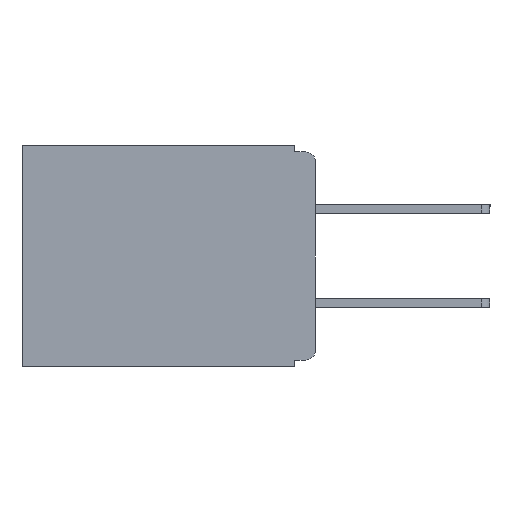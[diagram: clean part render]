
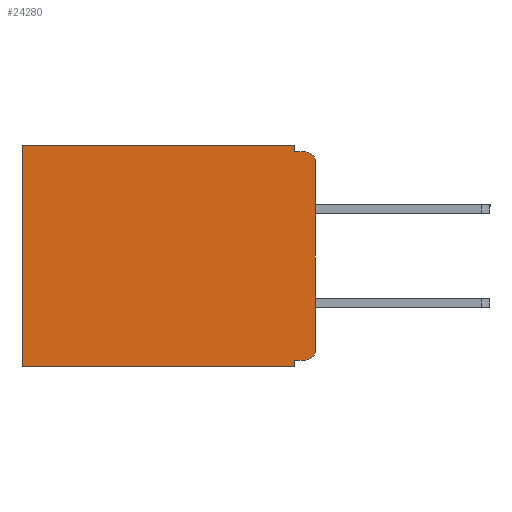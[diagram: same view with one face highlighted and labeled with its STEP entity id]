
A CAD part, left-side view. The second image highlights one B-rep face of the part: STEP entity #24280.
In plain terms, the highlighted planar face has unit normal (-1, 0, 0).
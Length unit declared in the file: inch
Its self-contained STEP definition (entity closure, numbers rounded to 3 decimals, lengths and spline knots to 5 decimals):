
#59 = VERTEX_POINT ( 'NONE', #13844 ) ;
#285 = DIRECTION ( 'NONE',  ( 0., 1., 0. ) ) ;
#644 = DIRECTION ( 'NONE',  ( 0., -1., 0. ) ) ;
#738 = DIRECTION ( 'NONE',  ( -1., 0., 0. ) ) ;
#985 = CARTESIAN_POINT ( 'NONE',  ( 0.3, 0.015, -0.01 ) ) ;
#1561 = DIRECTION ( 'NONE',  ( 0., 0., -1. ) ) ;
#1703 = CARTESIAN_POINT ( 'NONE',  ( 0.3, 0.015, -0.025 ) ) ;
#2041 = VERTEX_POINT ( 'NONE', #24072 ) ;
#2423 = AXIS2_PLACEMENT_3D ( 'NONE', #21740, #17787, #5472 ) ;
#2448 = CARTESIAN_POINT ( 'NONE',  ( 0.3, 0.031, 0. ) ) ;
#2542 = ORIENTED_EDGE ( 'NONE', *, *, #5101, .F. ) ;
#2576 = VERTEX_POINT ( 'NONE', #14432 ) ;
#3021 = EDGE_CURVE ( 'NONE', #2576, #8371, #4765, .T. ) ;
#3089 = CARTESIAN_POINT ( 'NONE',  ( 0.3, 0., 0. ) ) ;
#3917 = DIRECTION ( 'NONE',  ( 0., 0., -1. ) ) ;
#3938 = ORIENTED_EDGE ( 'NONE', *, *, #6344, .F. ) ;
#3987 = CARTESIAN_POINT ( 'NONE',  ( 0.3, 0., -0.33 ) ) ;
#4036 = EDGE_CURVE ( 'NONE', #5788, #26001, #7633, .T. ) ;
#4235 = ORIENTED_EDGE ( 'NONE', *, *, #3021, .F. ) ;
#4750 = ORIENTED_EDGE ( 'NONE', *, *, #4036, .T. ) ;
#4765 = LINE ( 'NONE', #9097, #25895 ) ;
#5101 = EDGE_CURVE ( 'NONE', #59, #2041, #20043, .T. ) ;
#5116 = ORIENTED_EDGE ( 'NONE', *, *, #23832, .T. ) ;
#5235 = DIRECTION ( 'NONE',  ( 0., 1., 0. ) ) ;
#5461 = CIRCLE ( 'NONE', #6372, 0.015 ) ;
#5472 = DIRECTION ( 'NONE',  ( 0., 0., -1. ) ) ;
#5529 = VECTOR ( 'NONE', #24273, 39.37008 ) ;
#5616 = ORIENTED_EDGE ( 'NONE', *, *, #23410, .F. ) ;
#5788 = VERTEX_POINT ( 'NONE', #26110 ) ;
#5924 = CARTESIAN_POINT ( 'NONE',  ( 0.3, 0.031, -0.33 ) ) ;
#6014 = ORIENTED_EDGE ( 'NONE', *, *, #14073, .T. ) ;
#6283 = ORIENTED_EDGE ( 'NONE', *, *, #7643, .T. ) ;
#6339 = ORIENTED_EDGE ( 'NONE', *, *, #14649, .F. ) ;
#6344 = EDGE_CURVE ( 'NONE', #5788, #2576, #7225, .T. ) ;
#6372 = AXIS2_PLACEMENT_3D ( 'NONE', #1703, #16302, #3917 ) ;
#6622 = ORIENTED_EDGE ( 'NONE', *, *, #25411, .F. ) ;
#7225 = LINE ( 'NONE', #2448, #13378 ) ;
#7633 = LINE ( 'NONE', #3089, #13754 ) ;
#7643 = EDGE_CURVE ( 'NONE', #19020, #2041, #12660, .T. ) ;
#7980 = VECTOR ( 'NONE', #5235, 39.37008 ) ;
#8069 = VECTOR ( 'NONE', #1561, 39.37008 ) ;
#8371 = VERTEX_POINT ( 'NONE', #985 ) ;
#8650 = LINE ( 'NONE', #11404, #7980 ) ;
#9097 = CARTESIAN_POINT ( 'NONE',  ( 0.3, 0., -0.01 ) ) ;
#9221 = VECTOR ( 'NONE', #9897, 39.37008 ) ;
#9897 = DIRECTION ( 'NONE',  ( 0., 0., -1. ) ) ;
#10332 = FACE_OUTER_BOUND ( 'NONE', #14225, .T. ) ;
#11075 = CARTESIAN_POINT ( 'NONE',  ( 0.3, 0.031, -0.32 ) ) ;
#11077 = LINE ( 'NONE', #14146, #5529 ) ;
#11404 = CARTESIAN_POINT ( 'NONE',  ( 0.3, 0., -0.32 ) ) ;
#11496 = VERTEX_POINT ( 'NONE', #11075 ) ;
#12199 = DIRECTION ( 'NONE',  ( 0., 1., 0. ) ) ;
#12660 = CIRCLE ( 'NONE', #14008, 0.015 ) ;
#12792 = CARTESIAN_POINT ( 'NONE',  ( 0.3, 0.015, -0.32 ) ) ;
#13124 = DIRECTION ( 'NONE',  ( 0., 0., -1. ) ) ;
#13362 = CARTESIAN_POINT ( 'NONE',  ( 0.3, 0.437, 0. ) ) ;
#13368 = CARTESIAN_POINT ( 'NONE',  ( 0.3, 0.015, -0.305 ) ) ;
#13378 = VECTOR ( 'NONE', #13124, 39.37008 ) ;
#13754 = VECTOR ( 'NONE', #12199, 39.37008 ) ;
#13844 = CARTESIAN_POINT ( 'NONE',  ( 0.3, 0., -0.025 ) ) ;
#14008 = AXIS2_PLACEMENT_3D ( 'NONE', #13368, #738, #15381 ) ;
#14073 = EDGE_CURVE ( 'NONE', #26001, #22040, #11077, .T. ) ;
#14146 = CARTESIAN_POINT ( 'NONE',  ( 0.3, 0.437, -0.33 ) ) ;
#14225 = EDGE_LOOP ( 'NONE', ( #2542, #5116, #4235, #3938, #4750, #6014, #5616, #6339, #6622, #6283 ) ) ;
#14432 = CARTESIAN_POINT ( 'NONE',  ( 0.3, 0.031, -0.01 ) ) ;
#14649 = EDGE_CURVE ( 'NONE', #11496, #24389, #24336, .T. ) ;
#15381 = DIRECTION ( 'NONE',  ( 0., 0., -1. ) ) ;
#15726 = PLANE ( 'NONE',  #2423 ) ;
#16165 = CARTESIAN_POINT ( 'NONE',  ( 0.3, 0.031, -0.33 ) ) ;
#16302 = DIRECTION ( 'NONE',  ( -1., 0., 0. ) ) ;
#17787 = DIRECTION ( 'NONE',  ( 1., 0., 0. ) ) ;
#19020 = VERTEX_POINT ( 'NONE', #12792 ) ;
#20043 = LINE ( 'NONE', #3987, #9221 ) ;
#20261 = CARTESIAN_POINT ( 'NONE',  ( 0.3, 0.437, -0.33 ) ) ;
#20540 = VECTOR ( 'NONE', #285, 39.37008 ) ;
#21740 = CARTESIAN_POINT ( 'NONE',  ( 0.3, 0., -0.33 ) ) ;
#21796 = LINE ( 'NONE', #25115, #20540 ) ;
#22040 = VERTEX_POINT ( 'NONE', #20261 ) ;
#23410 = EDGE_CURVE ( 'NONE', #24389, #22040, #21796, .T. ) ;
#23832 = EDGE_CURVE ( 'NONE', #59, #8371, #5461, .T. ) ;
#24072 = CARTESIAN_POINT ( 'NONE',  ( 0.3, 0., -0.305 ) ) ;
#24273 = DIRECTION ( 'NONE',  ( 0., 0., -1. ) ) ;
#24280 = ADVANCED_FACE ( 'NONE', ( #10332 ), #15726, .F. ) ;
#24336 = LINE ( 'NONE', #16165, #8069 ) ;
#24389 = VERTEX_POINT ( 'NONE', #5924 ) ;
#25115 = CARTESIAN_POINT ( 'NONE',  ( 0.3, 0., -0.33 ) ) ;
#25411 = EDGE_CURVE ( 'NONE', #19020, #11496, #8650, .T. ) ;
#25895 = VECTOR ( 'NONE', #644, 39.37008 ) ;
#26001 = VERTEX_POINT ( 'NONE', #13362 ) ;
#26110 = CARTESIAN_POINT ( 'NONE',  ( 0.3, 0.031, 0. ) ) ;
